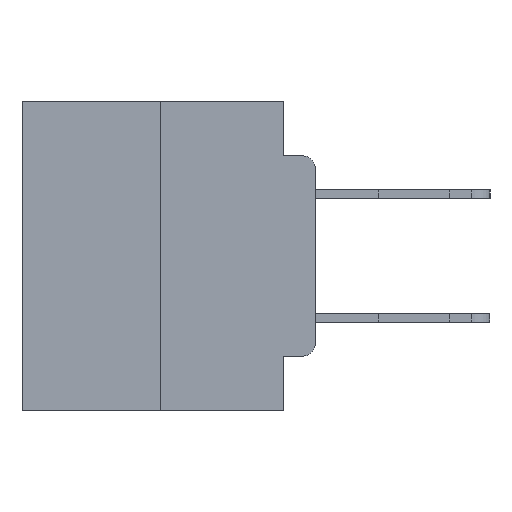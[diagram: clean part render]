
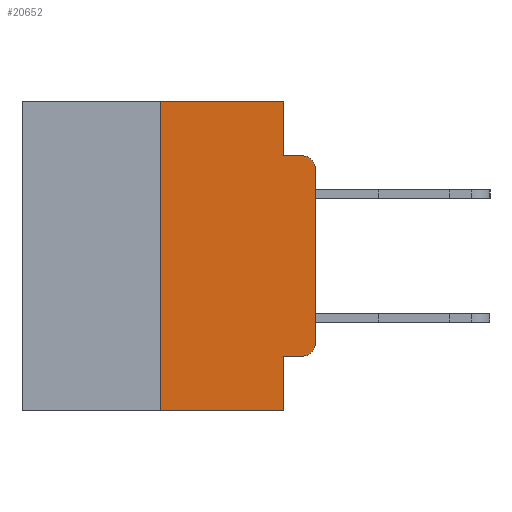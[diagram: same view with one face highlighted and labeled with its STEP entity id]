
A CAD part, left-side view. The second image highlights one B-rep face of the part: STEP entity #20652.
In plain terms, the highlighted planar face has unit normal (-1, 0, 0).
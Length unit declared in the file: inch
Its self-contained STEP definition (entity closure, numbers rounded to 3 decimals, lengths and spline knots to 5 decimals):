
#196 = LINE ( 'NONE', #11216, #22586 ) ;
#831 = ORIENTED_EDGE ( 'NONE', *, *, #13503, .T. ) ;
#1610 = DIRECTION ( 'NONE',  ( 0., -1., 0. ) ) ;
#1807 = ORIENTED_EDGE ( 'NONE', *, *, #18237, .F. ) ;
#1847 = DIRECTION ( 'NONE',  ( 0., -1., 0. ) ) ;
#1894 = EDGE_CURVE ( 'NONE', #20303, #4135, #14828, .T. ) ;
#2402 = CARTESIAN_POINT ( 'NONE',  ( 0., 0.051, 0. ) ) ;
#2647 = VERTEX_POINT ( 'NONE', #15301 ) ;
#3135 = CARTESIAN_POINT ( 'NONE',  ( 0., 0.473, 0. ) ) ;
#3841 = VECTOR ( 'NONE', #21254, 39.37008 ) ;
#4098 = CARTESIAN_POINT ( 'NONE',  ( 0., 0.25, 0. ) ) ;
#4131 = CARTESIAN_POINT ( 'NONE',  ( 0., 0.473, -0.5 ) ) ;
#4135 = VERTEX_POINT ( 'NONE', #13873 ) ;
#4145 = CARTESIAN_POINT ( 'NONE',  ( 0., 0.25, -0.5 ) ) ;
#4531 = CARTESIAN_POINT ( 'NONE',  ( 0., 0.02, -0.1085 ) ) ;
#4562 = LINE ( 'NONE', #25135, #26452 ) ;
#4787 = ORIENTED_EDGE ( 'NONE', *, *, #18114, .F. ) ;
#4975 = FACE_OUTER_BOUND ( 'NONE', #25051, .T. ) ;
#5063 = DIRECTION ( 'NONE',  ( 0., 0., -1. ) ) ;
#5296 = ORIENTED_EDGE ( 'NONE', *, *, #15428, .T. ) ;
#5398 = DIRECTION ( 'NONE',  ( 0., 0., -1. ) ) ;
#5698 = CARTESIAN_POINT ( 'NONE',  ( 0., 0., -0.3915 ) ) ;
#5751 = VECTOR ( 'NONE', #16418, 39.37008 ) ;
#6203 = EDGE_CURVE ( 'NONE', #7774, #10882, #24994, .T. ) ;
#6210 = ORIENTED_EDGE ( 'NONE', *, *, #22442, .F. ) ;
#6693 = VERTEX_POINT ( 'NONE', #18581 ) ;
#6755 = DIRECTION ( 'NONE',  ( 0., 0., -1. ) ) ;
#7221 = DIRECTION ( 'NONE',  ( -1., 0., 0. ) ) ;
#7676 = AXIS2_PLACEMENT_3D ( 'NONE', #3135, #18265, #5398 ) ;
#7684 = EDGE_CURVE ( 'NONE', #13708, #10882, #16096, .T. ) ;
#7774 = VERTEX_POINT ( 'NONE', #26976 ) ;
#8659 = DIRECTION ( 'NONE',  ( 0., 0., 1. ) ) ;
#9361 = LINE ( 'NONE', #20067, #10727 ) ;
#9543 = LINE ( 'NONE', #14421, #5751 ) ;
#9811 = ORIENTED_EDGE ( 'NONE', *, *, #16829, .T. ) ;
#10727 = VECTOR ( 'NONE', #5063, 39.37008 ) ;
#10882 = VERTEX_POINT ( 'NONE', #16035 ) ;
#11216 = CARTESIAN_POINT ( 'NONE',  ( 0., 0.473, 0. ) ) ;
#12434 = AXIS2_PLACEMENT_3D ( 'NONE', #4531, #19561, #6755 ) ;
#12468 = ORIENTED_EDGE ( 'NONE', *, *, #1894, .T. ) ;
#12484 = VECTOR ( 'NONE', #8659, 39.37008 ) ;
#12828 = DIRECTION ( 'NONE',  ( 0., -1., 0. ) ) ;
#13370 = DIRECTION ( 'NONE',  ( 0., -1., 0. ) ) ;
#13503 = EDGE_CURVE ( 'NONE', #25545, #13708, #22990, .T. ) ;
#13708 = VERTEX_POINT ( 'NONE', #24109 ) ;
#13873 = CARTESIAN_POINT ( 'NONE',  ( 0., 0.051, -0.5 ) ) ;
#13944 = ORIENTED_EDGE ( 'NONE', *, *, #6203, .F. ) ;
#14421 = CARTESIAN_POINT ( 'NONE',  ( 0., 0.051, 0. ) ) ;
#14828 = LINE ( 'NONE', #4131, #19733 ) ;
#15301 = CARTESIAN_POINT ( 'NONE',  ( 0., 0.02, -0.4115 ) ) ;
#15428 = EDGE_CURVE ( 'NONE', #2647, #25545, #27470, .T. ) ;
#16035 = CARTESIAN_POINT ( 'NONE',  ( 0., 0.02, -0.0885 ) ) ;
#16096 = CIRCLE ( 'NONE', #12434, 0.02 ) ;
#16418 = DIRECTION ( 'NONE',  ( 0., 0., -1. ) ) ;
#16829 = EDGE_CURVE ( 'NONE', #24075, #2647, #4562, .T. ) ;
#16973 = CARTESIAN_POINT ( 'NONE',  ( 0., 0.051, -0.0885 ) ) ;
#18111 = ORIENTED_EDGE ( 'NONE', *, *, #7684, .T. ) ;
#18114 = EDGE_CURVE ( 'NONE', #6693, #18164, #196, .T. ) ;
#18164 = VERTEX_POINT ( 'NONE', #2402 ) ;
#18237 = EDGE_CURVE ( 'NONE', #24075, #4135, #9361, .T. ) ;
#18265 = DIRECTION ( 'NONE',  ( 1., 0., 0. ) ) ;
#18581 = CARTESIAN_POINT ( 'NONE',  ( 0., 0.25, 0. ) ) ;
#19497 = VECTOR ( 'NONE', #12828, 39.37008 ) ;
#19561 = DIRECTION ( 'NONE',  ( -1., 0., 0. ) ) ;
#19733 = VECTOR ( 'NONE', #1847, 39.37008 ) ;
#20011 = CARTESIAN_POINT ( 'NONE',  ( 0., 0.02, -0.3915 ) ) ;
#20067 = CARTESIAN_POINT ( 'NONE',  ( 0., 0.051, 0. ) ) ;
#20303 = VERTEX_POINT ( 'NONE', #4145 ) ;
#20652 = ADVANCED_FACE ( 'NONE', ( #4975 ), #24423, .F. ) ;
#21254 = DIRECTION ( 'NONE',  ( 0., 0., 1. ) ) ;
#22100 = DIRECTION ( 'NONE',  ( 0., 0., -1. ) ) ;
#22442 = EDGE_CURVE ( 'NONE', #20303, #6693, #26447, .T. ) ;
#22586 = VECTOR ( 'NONE', #13370, 39.37008 ) ;
#22990 = LINE ( 'NONE', #23422, #12484 ) ;
#23422 = CARTESIAN_POINT ( 'NONE',  ( 0., 0., 0. ) ) ;
#24075 = VERTEX_POINT ( 'NONE', #24930 ) ;
#24109 = CARTESIAN_POINT ( 'NONE',  ( 0., 0., -0.1085 ) ) ;
#24423 = PLANE ( 'NONE',  #7676 ) ;
#24930 = CARTESIAN_POINT ( 'NONE',  ( 0., 0.051, -0.4115 ) ) ;
#24994 = LINE ( 'NONE', #16973, #19497 ) ;
#25051 = EDGE_LOOP ( 'NONE', ( #831, #18111, #13944, #25092, #4787, #6210, #12468, #1807, #9811, #5296 ) ) ;
#25092 = ORIENTED_EDGE ( 'NONE', *, *, #25186, .F. ) ;
#25135 = CARTESIAN_POINT ( 'NONE',  ( 0., 0.051, -0.4115 ) ) ;
#25186 = EDGE_CURVE ( 'NONE', #18164, #7774, #9543, .T. ) ;
#25545 = VERTEX_POINT ( 'NONE', #5698 ) ;
#26118 = AXIS2_PLACEMENT_3D ( 'NONE', #20011, #7221, #22100 ) ;
#26447 = LINE ( 'NONE', #4098, #3841 ) ;
#26452 = VECTOR ( 'NONE', #1610, 39.37008 ) ;
#26976 = CARTESIAN_POINT ( 'NONE',  ( 0., 0.051, -0.0885 ) ) ;
#27470 = CIRCLE ( 'NONE', #26118, 0.02 ) ;
